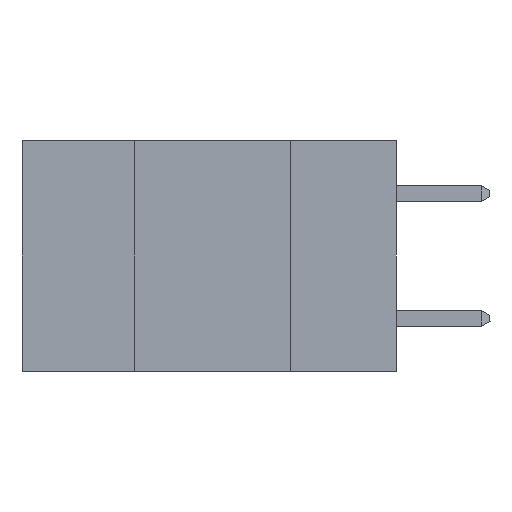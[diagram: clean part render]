
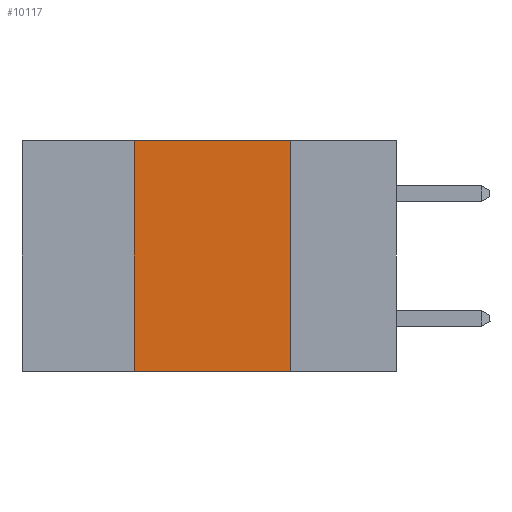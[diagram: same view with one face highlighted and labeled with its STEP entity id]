
A CAD part, left-side view. The second image highlights one B-rep face of the part: STEP entity #10117.
In plain terms, the highlighted planar face has unit normal (-1, 0, 0).
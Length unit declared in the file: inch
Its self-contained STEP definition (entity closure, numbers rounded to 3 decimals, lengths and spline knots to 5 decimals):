
#29 = ORIENTED_EDGE ( 'NONE', *, *, #6159, .F. ) ;
#265 = PLANE ( 'NONE',  #2895 ) ;
#392 = VECTOR ( 'NONE', #10629, 39.37008 ) ;
#720 = CARTESIAN_POINT ( 'NONE',  ( 0., 0.6, 0. ) ) ;
#939 = VECTOR ( 'NONE', #9587, 39.37008 ) ;
#1042 = ORIENTED_EDGE ( 'NONE', *, *, #10929, .F. ) ;
#1511 = VERTEX_POINT ( 'NONE', #6012 ) ;
#1642 = EDGE_CURVE ( 'NONE', #7470, #7396, #9243, .T. ) ;
#2059 = CARTESIAN_POINT ( 'NONE',  ( 0., 0.6, 0. ) ) ;
#2138 = EDGE_CURVE ( 'NONE', #7470, #1511, #6069, .T. ) ;
#2166 = CARTESIAN_POINT ( 'NONE',  ( 0., 0.17, -0.37 ) ) ;
#2333 = CARTESIAN_POINT ( 'NONE',  ( 0., 0.42, -0.37 ) ) ;
#2654 = CARTESIAN_POINT ( 'NONE',  ( 0., 0.6, -0.37 ) ) ;
#2895 = AXIS2_PLACEMENT_3D ( 'NONE', #2059, #4693, #8253 ) ;
#3045 = VECTOR ( 'NONE', #9029, 39.37008 ) ;
#3180 = DIRECTION ( 'NONE',  ( 0., -1., 0. ) ) ;
#3390 = CARTESIAN_POINT ( 'NONE',  ( 0., 0.42, -0.37 ) ) ;
#3544 = ORIENTED_EDGE ( 'NONE', *, *, #2138, .F. ) ;
#3677 = EDGE_LOOP ( 'NONE', ( #29, #1042, #3544, #4730 ) ) ;
#4693 = DIRECTION ( 'NONE',  ( 1., 0., 0. ) ) ;
#4730 = ORIENTED_EDGE ( 'NONE', *, *, #1642, .T. ) ;
#5413 = LINE ( 'NONE', #2166, #3045 ) ;
#5749 = FACE_OUTER_BOUND ( 'NONE', #3677, .T. ) ;
#6012 = CARTESIAN_POINT ( 'NONE',  ( 0., 0.42, 0. ) ) ;
#6069 = LINE ( 'NONE', #3390, #939 ) ;
#6159 = EDGE_CURVE ( 'NONE', #8452, #7396, #5413, .T. ) ;
#7396 = VERTEX_POINT ( 'NONE', #7399 ) ;
#7399 = CARTESIAN_POINT ( 'NONE',  ( 0., 0.17, -0.37 ) ) ;
#7410 = VECTOR ( 'NONE', #3180, 39.37008 ) ;
#7470 = VERTEX_POINT ( 'NONE', #2333 ) ;
#7558 = CARTESIAN_POINT ( 'NONE',  ( 0., 0.17, 0. ) ) ;
#8253 = DIRECTION ( 'NONE',  ( 0., 0., -1. ) ) ;
#8452 = VERTEX_POINT ( 'NONE', #7558 ) ;
#9029 = DIRECTION ( 'NONE',  ( 0., 0., -1. ) ) ;
#9243 = LINE ( 'NONE', #2654, #392 ) ;
#9587 = DIRECTION ( 'NONE',  ( 0., 0., 1. ) ) ;
#9713 = LINE ( 'NONE', #720, #7410 ) ;
#10117 = ADVANCED_FACE ( 'NONE', ( #5749 ), #265, .F. ) ;
#10629 = DIRECTION ( 'NONE',  ( 0., -1., 0. ) ) ;
#10929 = EDGE_CURVE ( 'NONE', #1511, #8452, #9713, .T. ) ;
